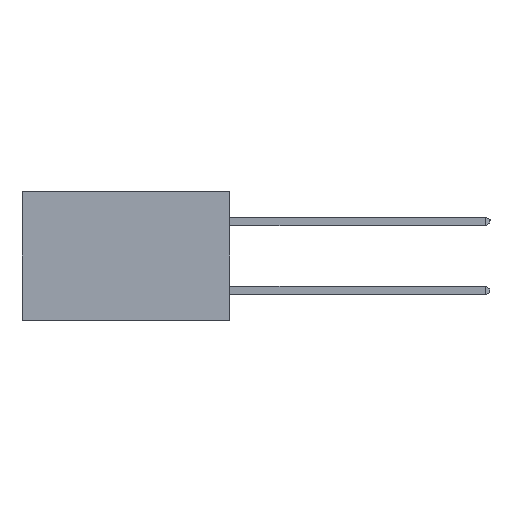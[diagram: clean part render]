
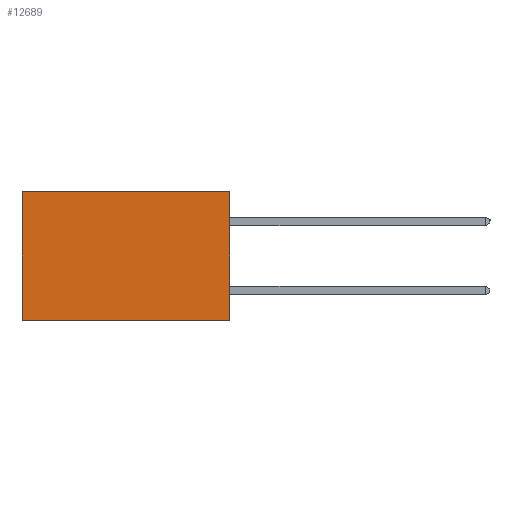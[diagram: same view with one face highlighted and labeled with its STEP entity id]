
A CAD part, left-side view. The second image highlights one B-rep face of the part: STEP entity #12689.
In plain terms, the highlighted planar face has unit normal (-1, 0, 0).
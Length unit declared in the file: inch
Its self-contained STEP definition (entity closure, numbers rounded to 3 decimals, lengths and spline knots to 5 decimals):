
#412 = DIRECTION ( 'NONE',  ( 0., 0., -1. ) ) ;
#709 = VERTEX_POINT ( 'NONE', #7465 ) ;
#1290 = LINE ( 'NONE', #10823, #13985 ) ;
#2182 = CARTESIAN_POINT ( 'NONE',  ( 0.298, 0.6, -0.37 ) ) ;
#3428 = VECTOR ( 'NONE', #17349, 39.37008 ) ;
#3499 = DIRECTION ( 'NONE',  ( 0., 0., -1. ) ) ;
#3815 = AXIS2_PLACEMENT_3D ( 'NONE', #16226, #9967, #412 ) ;
#4147 = DIRECTION ( 'NONE',  ( 0., 1., 0. ) ) ;
#4469 = CARTESIAN_POINT ( 'NONE',  ( 0.298, 0., 0. ) ) ;
#4572 = EDGE_CURVE ( 'NONE', #709, #10410, #16070, .T. ) ;
#4596 = LINE ( 'NONE', #8278, #12489 ) ;
#5208 = VERTEX_POINT ( 'NONE', #20051 ) ;
#5306 = LINE ( 'NONE', #4469, #16911 ) ;
#6711 = ORIENTED_EDGE ( 'NONE', *, *, #4572, .F. ) ;
#7391 = EDGE_CURVE ( 'NONE', #10273, #5208, #1290, .T. ) ;
#7465 = CARTESIAN_POINT ( 'NONE',  ( 0.298, 0., -0.37 ) ) ;
#7625 = EDGE_CURVE ( 'NONE', #10273, #709, #5306, .T. ) ;
#8278 = CARTESIAN_POINT ( 'NONE',  ( 0.298, 0.6, 0. ) ) ;
#8430 = CARTESIAN_POINT ( 'NONE',  ( 0.298, 0., -0.37 ) ) ;
#8932 = EDGE_CURVE ( 'NONE', #5208, #10410, #4596, .T. ) ;
#9967 = DIRECTION ( 'NONE',  ( 1., 0., 0. ) ) ;
#10273 = VERTEX_POINT ( 'NONE', #19258 ) ;
#10410 = VERTEX_POINT ( 'NONE', #2182 ) ;
#10823 = CARTESIAN_POINT ( 'NONE',  ( 0.298, 0., 0. ) ) ;
#11127 = DIRECTION ( 'NONE',  ( 0., 0., -1. ) ) ;
#11193 = ORIENTED_EDGE ( 'NONE', *, *, #7625, .F. ) ;
#12489 = VECTOR ( 'NONE', #3499, 39.37008 ) ;
#12689 = ADVANCED_FACE ( 'NONE', ( #16785 ), #19355, .F. ) ;
#13985 = VECTOR ( 'NONE', #4147, 39.37008 ) ;
#16070 = LINE ( 'NONE', #8430, #3428 ) ;
#16226 = CARTESIAN_POINT ( 'NONE',  ( 0.298, 0., 0. ) ) ;
#16785 = FACE_OUTER_BOUND ( 'NONE', #19117, .T. ) ;
#16911 = VECTOR ( 'NONE', #11127, 39.37008 ) ;
#17019 = ORIENTED_EDGE ( 'NONE', *, *, #7391, .T. ) ;
#17264 = ORIENTED_EDGE ( 'NONE', *, *, #8932, .T. ) ;
#17349 = DIRECTION ( 'NONE',  ( 0., 1., 0. ) ) ;
#19117 = EDGE_LOOP ( 'NONE', ( #17264, #6711, #11193, #17019 ) ) ;
#19258 = CARTESIAN_POINT ( 'NONE',  ( 0.298, 0., 0. ) ) ;
#19355 = PLANE ( 'NONE',  #3815 ) ;
#20051 = CARTESIAN_POINT ( 'NONE',  ( 0.298, 0.6, 0. ) ) ;
